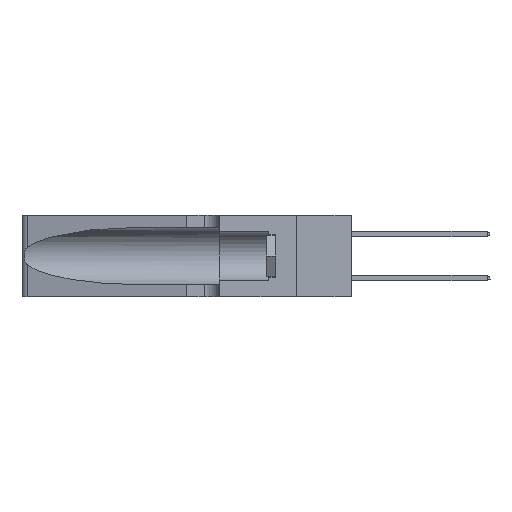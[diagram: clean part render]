
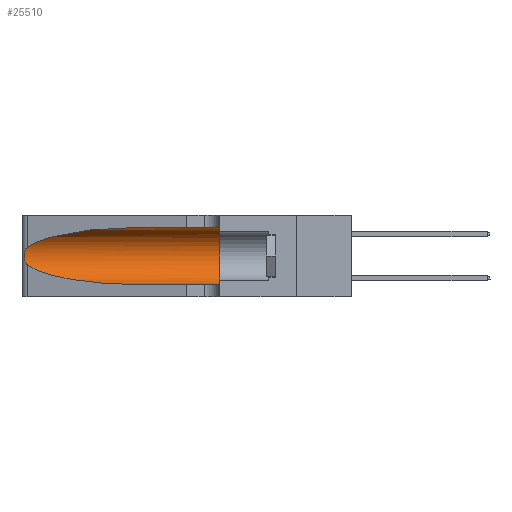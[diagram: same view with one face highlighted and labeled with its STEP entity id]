
A CAD part, left-side view. The second image highlights one B-rep face of the part: STEP entity #25510.
In plain terms, the highlighted cylindrical face has radius 3.308 mm (diameter 6.617 mm), a partial arc.
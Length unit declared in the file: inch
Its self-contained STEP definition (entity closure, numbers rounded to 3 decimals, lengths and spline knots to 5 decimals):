
#481 = CARTESIAN_POINT ( 'NONE',  ( 0.25487, 1.22718, 0.22369 ) ) ;
#1559 = ORIENTED_EDGE ( 'NONE', *, *, #27213, .F. ) ;
#2876 =( BOUNDED_CURVE ( )  B_SPLINE_CURVE ( 3, ( #24262, #22056, #9304, #24626 ),
 .UNSPECIFIED., .F., .T. ) 
 B_SPLINE_CURVE_WITH_KNOTS ( ( 4, 4 ),
 ( 1.5708, 2.84003 ),
 .UNSPECIFIED. ) 
 CURVE ( )  GEOMETRIC_REPRESENTATION_ITEM ( )  RATIONAL_B_SPLINE_CURVE ( ( 1., 0.87, 0.87, 1. ) ) 
 REPRESENTATION_ITEM ( '' )  );
#3114 = LINE ( 'NONE', #15594, #30407 ) ;
#3693 = CARTESIAN_POINT ( 'NONE',  ( 0.25639, 1.23184, 0.21858 ) ) ;
#4471 = DIRECTION ( 'NONE',  ( 0., 0., 1. ) ) ;
#6007 = EDGE_CURVE ( 'NONE', #30808, #9700, #9082, .T. ) ;
#6274 = CARTESIAN_POINT ( 'NONE',  ( 0.25487, 1.22718, 0.14631 ) ) ;
#6836 = CARTESIAN_POINT ( 'NONE',  ( 0.25487, 1.22718, 0.14631 ) ) ;
#7526 = CARTESIAN_POINT ( 'NONE',  ( 0.1305, 1.61858, 0.05475 ) ) ;
#7683 = CARTESIAN_POINT ( 'NONE',  ( 0.26075, 1.23896, 0.19203 ) ) ;
#8104 = LINE ( 'NONE', #7526, #18838 ) ;
#8178 = AXIS2_PLACEMENT_3D ( 'NONE', #21380, #25971, #10654 ) ;
#8899 = VERTEX_POINT ( 'NONE', #18221 ) ;
#8926 = CARTESIAN_POINT ( 'NONE',  ( 0.1305, 0.72297, 0.31525 ) ) ;
#9082 = CIRCLE ( 'NONE', #29468, 0.13025 ) ;
#9304 = CARTESIAN_POINT ( 'NONE',  ( 0.2373, 1.15595, 0.28018 ) ) ;
#9700 = VERTEX_POINT ( 'NONE', #20805 ) ;
#9914 = B_SPLINE_CURVE_WITH_KNOTS ( 'NONE', 3,
 ( #481, #27147, #3693, #31429, #31280, #29285, #7683, #10640, #17611, #28750, #28837, #32419, #26466, #29960 ),
 .UNSPECIFIED., .F., .F.,
 ( 4, 2, 2, 2, 2, 2, 4 ),
 ( 0., 0.00027, 0.00053, 0.00107, 0.0016, 0.00187, 0.00214 ),
 .UNSPECIFIED. ) ;
#9937 = CARTESIAN_POINT ( 'NONE',  ( 0.1305, 0.35, 0.31525 ) ) ;
#10640 = CARTESIAN_POINT ( 'NONE',  ( 0.26075, 1.23896, 0.178 ) ) ;
#10654 = DIRECTION ( 'NONE',  ( 0., 0., -1. ) ) ;
#11372 = VERTEX_POINT ( 'NONE', #6274 ) ;
#12224 = CARTESIAN_POINT ( 'NONE',  ( 0.18966, 0.96281, 0.05475 ) ) ;
#12259 = ORIENTED_EDGE ( 'NONE', *, *, #24244, .T. ) ;
#14565 = CARTESIAN_POINT ( 'NONE',  ( 0.2373, 1.15595, 0.08982 ) ) ;
#15594 = CARTESIAN_POINT ( 'NONE',  ( 0.1305, 1.61858, 0.31525 ) ) ;
#16391 =( BOUNDED_CURVE ( )  B_SPLINE_CURVE ( 3, ( #6836, #14565, #12224, #32477 ),
 .UNSPECIFIED., .F., .T. ) 
 B_SPLINE_CURVE_WITH_KNOTS ( ( 4, 4 ),
 ( 3.44316, 4.71239 ),
 .UNSPECIFIED. ) 
 CURVE ( )  GEOMETRIC_REPRESENTATION_ITEM ( )  RATIONAL_B_SPLINE_CURVE ( ( 1., 0.87, 0.87, 1. ) ) 
 REPRESENTATION_ITEM ( '' )  );
#17611 = CARTESIAN_POINT ( 'NONE',  ( 0.26017, 1.23833, 0.17102 ) ) ;
#17863 = DIRECTION ( 'NONE',  ( 0., -1., 0. ) ) ;
#18220 = VERTEX_POINT ( 'NONE', #28025 ) ;
#18221 = CARTESIAN_POINT ( 'NONE',  ( 0.25487, 1.22718, 0.22369 ) ) ;
#18838 = VECTOR ( 'NONE', #20672, 39.37008 ) ;
#20158 = CARTESIAN_POINT ( 'NONE',  ( 0.1305, 0.35, 0.185 ) ) ;
#20672 = DIRECTION ( 'NONE',  ( 0., -1., 0. ) ) ;
#20805 = CARTESIAN_POINT ( 'NONE',  ( 0.1305, 0.35, 0.05475 ) ) ;
#21380 = CARTESIAN_POINT ( 'NONE',  ( 0.1305, 1.61858, 0.185 ) ) ;
#21423 = EDGE_CURVE ( 'NONE', #32622, #8899, #2876, .T. ) ;
#22056 = CARTESIAN_POINT ( 'NONE',  ( 0.18966, 0.96281, 0.31525 ) ) ;
#23338 = EDGE_CURVE ( 'NONE', #8899, #11372, #9914, .T. ) ;
#24244 = EDGE_CURVE ( 'NONE', #11372, #18220, #16391, .T. ) ;
#24262 = CARTESIAN_POINT ( 'NONE',  ( 0.1305, 0.72297, 0.31525 ) ) ;
#24626 = CARTESIAN_POINT ( 'NONE',  ( 0.25487, 1.22718, 0.22369 ) ) ;
#24836 = EDGE_CURVE ( 'NONE', #18220, #9700, #8104, .T. ) ;
#25189 = ORIENTED_EDGE ( 'NONE', *, *, #23338, .T. ) ;
#25510 = ADVANCED_FACE ( 'NONE', ( #27254 ), #28438, .F. ) ;
#25971 = DIRECTION ( 'NONE',  ( 0., -1., 0. ) ) ;
#26466 = CARTESIAN_POINT ( 'NONE',  ( 0.25555, 1.22993, 0.14849 ) ) ;
#27147 = CARTESIAN_POINT ( 'NONE',  ( 0.25555, 1.22994, 0.2215 ) ) ;
#27213 = EDGE_CURVE ( 'NONE', #32622, #30808, #3114, .T. ) ;
#27254 = FACE_OUTER_BOUND ( 'NONE', #28869, .T. ) ;
#27418 = DIRECTION ( 'NONE',  ( 0., 1., 0. ) ) ;
#28025 = CARTESIAN_POINT ( 'NONE',  ( 0.1305, 0.72297, 0.05475 ) ) ;
#28259 = ORIENTED_EDGE ( 'NONE', *, *, #6007, .F. ) ;
#28438 = CYLINDRICAL_SURFACE ( 'NONE', #8178, 0.13025 ) ;
#28750 = CARTESIAN_POINT ( 'NONE',  ( 0.25856, 1.23593, 0.16098 ) ) ;
#28837 = CARTESIAN_POINT ( 'NONE',  ( 0.25789, 1.23486, 0.15765 ) ) ;
#28869 = EDGE_LOOP ( 'NONE', ( #32273, #25189, #12259, #31892, #28259, #1559 ) ) ;
#29285 = CARTESIAN_POINT ( 'NONE',  ( 0.26018, 1.23835, 0.19895 ) ) ;
#29468 = AXIS2_PLACEMENT_3D ( 'NONE', #20158, #27418, #4471 ) ;
#29960 = CARTESIAN_POINT ( 'NONE',  ( 0.25487, 1.22718, 0.14631 ) ) ;
#30407 = VECTOR ( 'NONE', #17863, 39.37008 ) ;
#30808 = VERTEX_POINT ( 'NONE', #9937 ) ;
#31280 = CARTESIAN_POINT ( 'NONE',  ( 0.25854, 1.2359, 0.20912 ) ) ;
#31429 = CARTESIAN_POINT ( 'NONE',  ( 0.25787, 1.23484, 0.2124 ) ) ;
#31892 = ORIENTED_EDGE ( 'NONE', *, *, #24836, .T. ) ;
#32273 = ORIENTED_EDGE ( 'NONE', *, *, #21423, .T. ) ;
#32419 = CARTESIAN_POINT ( 'NONE',  ( 0.25639, 1.23186, 0.15144 ) ) ;
#32477 = CARTESIAN_POINT ( 'NONE',  ( 0.1305, 0.72297, 0.05475 ) ) ;
#32622 = VERTEX_POINT ( 'NONE', #8926 ) ;
